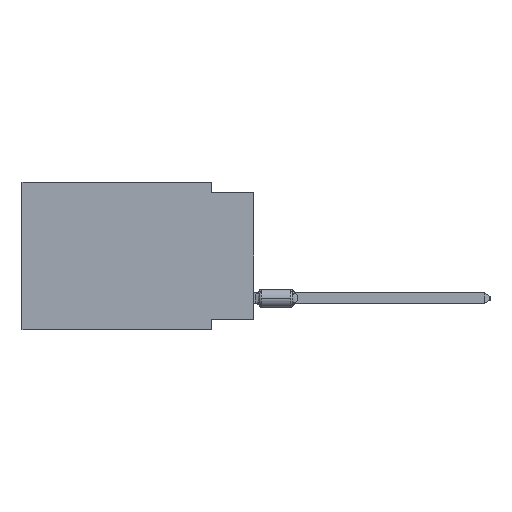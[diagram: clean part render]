
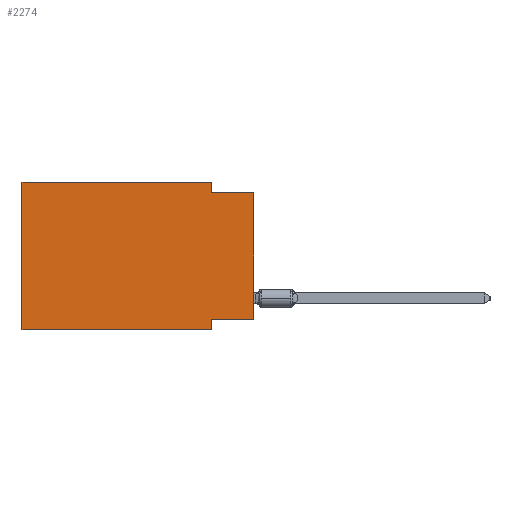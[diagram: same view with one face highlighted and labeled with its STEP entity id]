
A CAD part, left-side view. The second image highlights one B-rep face of the part: STEP entity #2274.
In plain terms, the highlighted planar face has unit normal (-1, 0, 0).
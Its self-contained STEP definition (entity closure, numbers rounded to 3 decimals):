
#1031 = DIRECTION ( 'NONE',  ( 0., -1., 0. ) ) ;
#1274 = ORIENTED_EDGE ( 'NONE', *, *, #33859, .T. ) ;
#1333 = VECTOR ( 'NONE', #25845, 1000. ) ;
#1693 = CARTESIAN_POINT ( 'NONE',  ( 0., 13.97, -8.89 ) ) ;
#2274 = ADVANCED_FACE ( 'NONE', ( #22377 ), #12600, .F. ) ;
#4834 = EDGE_CURVE ( 'NONE', #36273, #5423, #41371, .T. ) ;
#5423 = VERTEX_POINT ( 'NONE', #33306 ) ;
#5477 = CARTESIAN_POINT ( 'NONE',  ( 0., 2.54, -0.635 ) ) ;
#5940 = ORIENTED_EDGE ( 'NONE', *, *, #20780, .F. ) ;
#6101 = ORIENTED_EDGE ( 'NONE', *, *, #52095, .F. ) ;
#7396 = CARTESIAN_POINT ( 'NONE',  ( 0., 0., -8.255 ) ) ;
#8084 = CARTESIAN_POINT ( 'NONE',  ( 0., 13.97, 0. ) ) ;
#10379 = VECTOR ( 'NONE', #46238, 1000. ) ;
#10832 = DIRECTION ( 'NONE',  ( 0., -1., 0. ) ) ;
#10939 = VECTOR ( 'NONE', #21272, 1000. ) ;
#11675 = VERTEX_POINT ( 'NONE', #35391 ) ;
#11697 = VERTEX_POINT ( 'NONE', #41170 ) ;
#12237 = AXIS2_PLACEMENT_3D ( 'NONE', #16893, #48861, #58292 ) ;
#12600 = PLANE ( 'NONE',  #12237 ) ;
#12719 = CARTESIAN_POINT ( 'NONE',  ( 0., 0., -0.635 ) ) ;
#14400 = ORIENTED_EDGE ( 'NONE', *, *, #45383, .F. ) ;
#14674 = VECTOR ( 'NONE', #23705, 1000. ) ;
#16893 = CARTESIAN_POINT ( 'NONE',  ( 0., 13.97, 0. ) ) ;
#20780 = EDGE_CURVE ( 'NONE', #11697, #11675, #38009, .T. ) ;
#21272 = DIRECTION ( 'NONE',  ( 0., 0., 1. ) ) ;
#21476 = VERTEX_POINT ( 'NONE', #7396 ) ;
#22377 = FACE_OUTER_BOUND ( 'NONE', #57837, .T. ) ;
#23705 = DIRECTION ( 'NONE',  ( 0., 0., -1. ) ) ;
#24246 = EDGE_CURVE ( 'NONE', #59660, #53000, #53248, .T. ) ;
#25845 = DIRECTION ( 'NONE',  ( 0., 0., -1. ) ) ;
#26135 = CARTESIAN_POINT ( 'NONE',  ( 0., 2.54, 0. ) ) ;
#26313 = ORIENTED_EDGE ( 'NONE', *, *, #31563, .F. ) ;
#26578 = ORIENTED_EDGE ( 'NONE', *, *, #4834, .F. ) ;
#26954 = DIRECTION ( 'NONE',  ( 0., 1., 0. ) ) ;
#27562 = CARTESIAN_POINT ( 'NONE',  ( 0., 0., -8.255 ) ) ;
#27611 = DIRECTION ( 'NONE',  ( 0., -1., 0. ) ) ;
#30005 = VERTEX_POINT ( 'NONE', #12719 ) ;
#31563 = EDGE_CURVE ( 'NONE', #21476, #11697, #55256, .T. ) ;
#32851 = CARTESIAN_POINT ( 'NONE',  ( 0., 2.54, -8.89 ) ) ;
#33306 = CARTESIAN_POINT ( 'NONE',  ( 0., 13.97, 0. ) ) ;
#33824 = VECTOR ( 'NONE', #27611, 1000. ) ;
#33859 = EDGE_CURVE ( 'NONE', #21476, #30005, #45002, .T. ) ;
#33944 = CARTESIAN_POINT ( 'NONE',  ( 0., 13.97, -8.89 ) ) ;
#35391 = CARTESIAN_POINT ( 'NONE',  ( 0., 2.54, -8.89 ) ) ;
#35567 = CARTESIAN_POINT ( 'NONE',  ( 0., 0., 0. ) ) ;
#36273 = VERTEX_POINT ( 'NONE', #1693 ) ;
#36500 = CARTESIAN_POINT ( 'NONE',  ( 0., 13.97, 0. ) ) ;
#38009 = LINE ( 'NONE', #32851, #14674 ) ;
#38843 = CARTESIAN_POINT ( 'NONE',  ( 0., 0., -0.635 ) ) ;
#41170 = CARTESIAN_POINT ( 'NONE',  ( 0., 2.54, -8.255 ) ) ;
#41371 = LINE ( 'NONE', #36500, #10379 ) ;
#42681 = EDGE_CURVE ( 'NONE', #36273, #11675, #51590, .T. ) ;
#45002 = LINE ( 'NONE', #35567, #10939 ) ;
#45383 = EDGE_CURVE ( 'NONE', #53000, #30005, #57118, .T. ) ;
#46238 = DIRECTION ( 'NONE',  ( 0., 0., 1. ) ) ;
#46478 = LINE ( 'NONE', #8084, #33824 ) ;
#47187 = VECTOR ( 'NONE', #1031, 1000. ) ;
#48861 = DIRECTION ( 'NONE',  ( 1., 0., 0. ) ) ;
#51212 = ORIENTED_EDGE ( 'NONE', *, *, #24246, .F. ) ;
#51590 = LINE ( 'NONE', #33944, #47187 ) ;
#52095 = EDGE_CURVE ( 'NONE', #5423, #59660, #46478, .T. ) ;
#53000 = VERTEX_POINT ( 'NONE', #5477 ) ;
#53248 = LINE ( 'NONE', #26135, #1333 ) ;
#53624 = ORIENTED_EDGE ( 'NONE', *, *, #42681, .T. ) ;
#55256 = LINE ( 'NONE', #27562, #57004 ) ;
#57004 = VECTOR ( 'NONE', #26954, 1000. ) ;
#57118 = LINE ( 'NONE', #38843, #58264 ) ;
#57447 = CARTESIAN_POINT ( 'NONE',  ( 0., 2.54, 0. ) ) ;
#57837 = EDGE_LOOP ( 'NONE', ( #1274, #14400, #51212, #6101, #26578, #53624, #5940, #26313 ) ) ;
#58264 = VECTOR ( 'NONE', #10832, 1000. ) ;
#58292 = DIRECTION ( 'NONE',  ( 0., 0., -1. ) ) ;
#59660 = VERTEX_POINT ( 'NONE', #57447 ) ;
